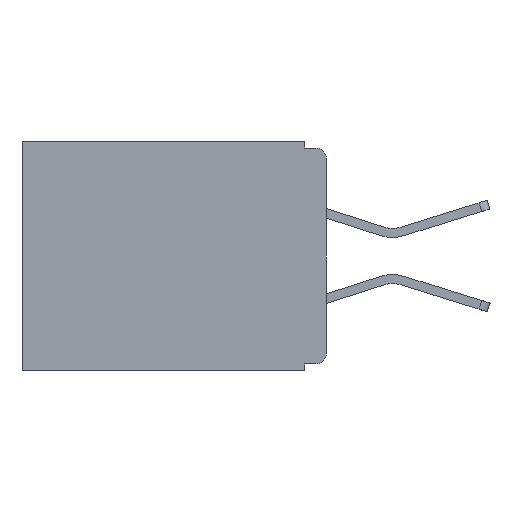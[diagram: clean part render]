
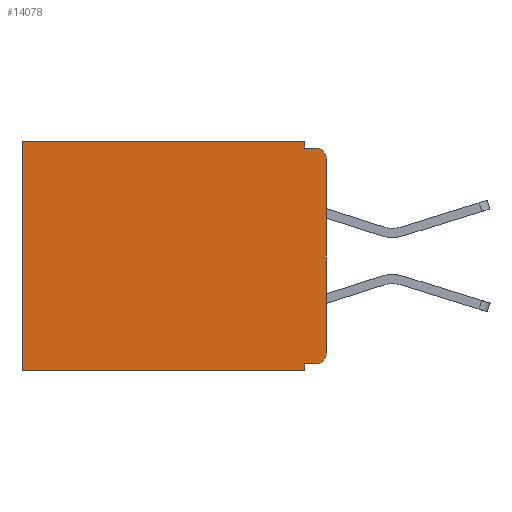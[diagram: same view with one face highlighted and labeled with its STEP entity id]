
A CAD part, left-side view. The second image highlights one B-rep face of the part: STEP entity #14078.
In plain terms, the highlighted planar face has unit normal (-1, 0, 0).
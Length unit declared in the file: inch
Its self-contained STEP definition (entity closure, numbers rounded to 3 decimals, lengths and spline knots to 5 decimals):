
#185 = ORIENTED_EDGE ( 'NONE', *, *, #17979, .F. ) ;
#281 = DIRECTION ( 'NONE',  ( 0., 0., -1. ) ) ;
#526 = ORIENTED_EDGE ( 'NONE', *, *, #3920, .T. ) ;
#643 = DIRECTION ( 'NONE',  ( 0., 1., 0. ) ) ;
#761 = CARTESIAN_POINT ( 'NONE',  ( 0.3, 0., -0.32 ) ) ;
#1233 = CARTESIAN_POINT ( 'NONE',  ( 0.3, 0.031, 0. ) ) ;
#1830 = DIRECTION ( 'NONE',  ( 0., 1., 0. ) ) ;
#2173 = CARTESIAN_POINT ( 'NONE',  ( 0.3, 0.015, -0.305 ) ) ;
#2746 = EDGE_CURVE ( 'NONE', #28325, #27208, #19125, .T. ) ;
#3675 = VECTOR ( 'NONE', #643, 39.37008 ) ;
#3682 = CARTESIAN_POINT ( 'NONE',  ( 0.3, 0., -0.33 ) ) ;
#3920 = EDGE_CURVE ( 'NONE', #26774, #26747, #5430, .T. ) ;
#4190 = CARTESIAN_POINT ( 'NONE',  ( 0.3, 0.031, -0.32 ) ) ;
#4767 = DIRECTION ( 'NONE',  ( 0., 0., -1. ) ) ;
#5385 = ORIENTED_EDGE ( 'NONE', *, *, #12872, .T. ) ;
#5430 = LINE ( 'NONE', #30720, #31126 ) ;
#5532 = VECTOR ( 'NONE', #1830, 39.37008 ) ;
#6003 = CARTESIAN_POINT ( 'NONE',  ( 0.3, 0., -0.01 ) ) ;
#6053 = CARTESIAN_POINT ( 'NONE',  ( 0.3, 0.015, -0.32 ) ) ;
#6354 = VERTEX_POINT ( 'NONE', #1233 ) ;
#6843 = DIRECTION ( 'NONE',  ( 0., 1., 0. ) ) ;
#8082 = LINE ( 'NONE', #12841, #13320 ) ;
#8611 = DIRECTION ( 'NONE',  ( 0., -1., 0. ) ) ;
#8747 = VECTOR ( 'NONE', #8611, 39.37008 ) ;
#8783 = VECTOR ( 'NONE', #12239, 39.37008 ) ;
#8833 = EDGE_CURVE ( 'NONE', #10630, #25992, #17388, .T. ) ;
#9227 = ORIENTED_EDGE ( 'NONE', *, *, #8833, .F. ) ;
#9269 = CARTESIAN_POINT ( 'NONE',  ( 0.3, 0.015, -0.01 ) ) ;
#9544 = LINE ( 'NONE', #6003, #8747 ) ;
#10376 = LINE ( 'NONE', #24697, #8783 ) ;
#10630 = VERTEX_POINT ( 'NONE', #6053 ) ;
#11878 = FACE_OUTER_BOUND ( 'NONE', #20022, .T. ) ;
#12239 = DIRECTION ( 'NONE',  ( 0., 0., -1. ) ) ;
#12841 = CARTESIAN_POINT ( 'NONE',  ( 0.3, 0.031, 0. ) ) ;
#12872 = EDGE_CURVE ( 'NONE', #10630, #21319, #31944, .T. ) ;
#12953 = DIRECTION ( 'NONE',  ( 0., 0., -1. ) ) ;
#13235 = EDGE_CURVE ( 'NONE', #25289, #27208, #9544, .T. ) ;
#13320 = VECTOR ( 'NONE', #12953, 39.37008 ) ;
#13328 = LINE ( 'NONE', #3682, #19287 ) ;
#13624 = CARTESIAN_POINT ( 'NONE',  ( 0.3, 0.031, -0.33 ) ) ;
#14078 = ADVANCED_FACE ( 'NONE', ( #11878 ), #27263, .F. ) ;
#14215 = CARTESIAN_POINT ( 'NONE',  ( 0.3, 0., -0.305 ) ) ;
#14403 = VERTEX_POINT ( 'NONE', #13624 ) ;
#14532 = AXIS2_PLACEMENT_3D ( 'NONE', #2173, #20107, #4767 ) ;
#14534 = CARTESIAN_POINT ( 'NONE',  ( 0.3, 0., -0.33 ) ) ;
#14742 = CARTESIAN_POINT ( 'NONE',  ( 0.3, 0., 0. ) ) ;
#15013 = DIRECTION ( 'NONE',  ( 0., 0., -1. ) ) ;
#15323 = ORIENTED_EDGE ( 'NONE', *, *, #2746, .T. ) ;
#16292 = EDGE_CURVE ( 'NONE', #14403, #26747, #29967, .T. ) ;
#17073 = VECTOR ( 'NONE', #6843, 39.37008 ) ;
#17388 = LINE ( 'NONE', #761, #3675 ) ;
#17459 = CARTESIAN_POINT ( 'NONE',  ( 0.3, 0., -0.33 ) ) ;
#17979 = EDGE_CURVE ( 'NONE', #28325, #21319, #13328, .T. ) ;
#19060 = DIRECTION ( 'NONE',  ( 0., 0., -1. ) ) ;
#19125 = CIRCLE ( 'NONE', #30877, 0.015 ) ;
#19183 = ORIENTED_EDGE ( 'NONE', *, *, #16292, .F. ) ;
#19287 = VECTOR ( 'NONE', #28682, 39.37008 ) ;
#20022 = EDGE_LOOP ( 'NONE', ( #185, #15323, #25348, #29166, #20604, #526, #19183, #30987, #9227, #5385 ) ) ;
#20107 = DIRECTION ( 'NONE',  ( -1., 0., 0. ) ) ;
#20604 = ORIENTED_EDGE ( 'NONE', *, *, #25402, .T. ) ;
#21319 = VERTEX_POINT ( 'NONE', #14215 ) ;
#23673 = AXIS2_PLACEMENT_3D ( 'NONE', #17459, #29633, #15013 ) ;
#24090 = EDGE_CURVE ( 'NONE', #25992, #14403, #10376, .T. ) ;
#24697 = CARTESIAN_POINT ( 'NONE',  ( 0.3, 0.031, -0.33 ) ) ;
#25218 = CARTESIAN_POINT ( 'NONE',  ( 0.3, 0.437, 0. ) ) ;
#25289 = VERTEX_POINT ( 'NONE', #26283 ) ;
#25348 = ORIENTED_EDGE ( 'NONE', *, *, #13235, .F. ) ;
#25402 = EDGE_CURVE ( 'NONE', #6354, #26774, #25684, .T. ) ;
#25684 = LINE ( 'NONE', #14742, #5532 ) ;
#25992 = VERTEX_POINT ( 'NONE', #4190 ) ;
#26181 = CARTESIAN_POINT ( 'NONE',  ( 0.3, 0., -0.025 ) ) ;
#26283 = CARTESIAN_POINT ( 'NONE',  ( 0.3, 0.031, -0.01 ) ) ;
#26747 = VERTEX_POINT ( 'NONE', #29829 ) ;
#26774 = VERTEX_POINT ( 'NONE', #25218 ) ;
#27208 = VERTEX_POINT ( 'NONE', #9269 ) ;
#27220 = DIRECTION ( 'NONE',  ( -1., 0., 0. ) ) ;
#27263 = PLANE ( 'NONE',  #23673 ) ;
#28325 = VERTEX_POINT ( 'NONE', #26181 ) ;
#28682 = DIRECTION ( 'NONE',  ( 0., 0., -1. ) ) ;
#29166 = ORIENTED_EDGE ( 'NONE', *, *, #30515, .F. ) ;
#29391 = CARTESIAN_POINT ( 'NONE',  ( 0.3, 0.015, -0.025 ) ) ;
#29633 = DIRECTION ( 'NONE',  ( 1., 0., 0. ) ) ;
#29829 = CARTESIAN_POINT ( 'NONE',  ( 0.3, 0.437, -0.33 ) ) ;
#29967 = LINE ( 'NONE', #14534, #17073 ) ;
#30515 = EDGE_CURVE ( 'NONE', #6354, #25289, #8082, .T. ) ;
#30720 = CARTESIAN_POINT ( 'NONE',  ( 0.3, 0.437, -0.33 ) ) ;
#30877 = AXIS2_PLACEMENT_3D ( 'NONE', #29391, #27220, #281 ) ;
#30987 = ORIENTED_EDGE ( 'NONE', *, *, #24090, .F. ) ;
#31126 = VECTOR ( 'NONE', #19060, 39.37008 ) ;
#31944 = CIRCLE ( 'NONE', #14532, 0.015 ) ;
